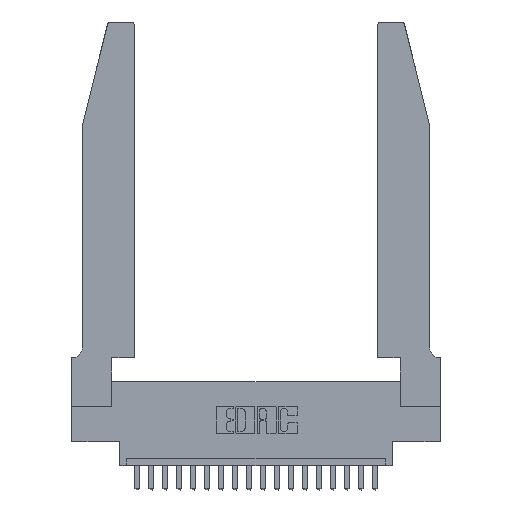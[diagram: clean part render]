
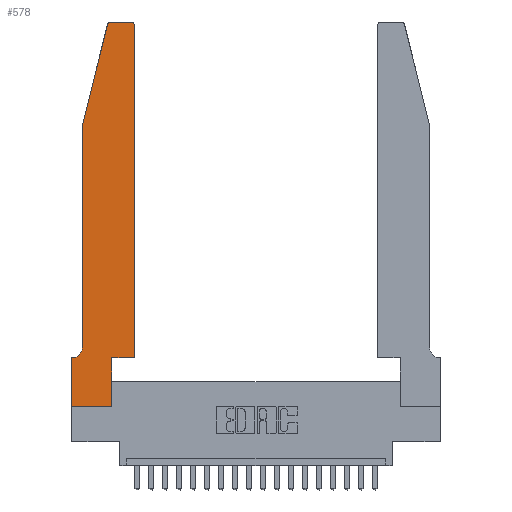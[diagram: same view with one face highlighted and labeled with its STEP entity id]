
A CAD part, top view. The second image highlights one B-rep face of the part: STEP entity #578.
In plain terms, the highlighted planar face has unit normal (0, 0, 1).
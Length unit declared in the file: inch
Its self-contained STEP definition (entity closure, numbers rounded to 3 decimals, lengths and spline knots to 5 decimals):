
#219 = CARTESIAN_POINT ( 'NONE',  ( 0.25487, 2.72718, 0.37 ) ) ;
#357 = LINE ( 'NONE', #1117, #12515 ) ;
#433 = AXIS2_PLACEMENT_3D ( 'NONE', #7943, #5994, #16182 ) ;
#545 = ORIENTED_EDGE ( 'NONE', *, *, #14522, .T. ) ;
#578 = ADVANCED_FACE ( 'NONE', ( #14978 ), #3425, .T. ) ;
#1117 = CARTESIAN_POINT ( 'NONE',  ( 0., 0., 0.37 ) ) ;
#1259 = DIRECTION ( 'NONE',  ( 1., 0., 0. ) ) ;
#1441 = LINE ( 'NONE', #11707, #9361 ) ;
#1527 = EDGE_CURVE ( 'NONE', #6507, #6493, #13141, .T. ) ;
#1722 = CARTESIAN_POINT ( 'NONE',  ( 0., 0.35, 0.37 ) ) ;
#2062 = EDGE_CURVE ( 'NONE', #17712, #14820, #6023, .T. ) ;
#2154 = ORIENTED_EDGE ( 'NONE', *, *, #14371, .T. ) ;
#2862 = CARTESIAN_POINT ( 'NONE',  ( 0.0755, 2., 0.37 ) ) ;
#3166 = VERTEX_POINT ( 'NONE', #11669 ) ;
#3185 = LINE ( 'NONE', #8729, #4270 ) ;
#3213 = CARTESIAN_POINT ( 'NONE',  ( 0.0055, 0.35, 0.37 ) ) ;
#3301 = VECTOR ( 'NONE', #17270, 39.37008 ) ;
#3425 = PLANE ( 'NONE',  #14117 ) ;
#3438 = CARTESIAN_POINT ( 'NONE',  ( 0.284, 2.75, 0.37 ) ) ;
#4258 = CARTESIAN_POINT ( 'NONE',  ( 0.2865, 0.35, 0.37 ) ) ;
#4270 = VECTOR ( 'NONE', #5372, 39.37008 ) ;
#4345 = CIRCLE ( 'NONE', #5664, 0.03 ) ;
#4473 = EDGE_CURVE ( 'NONE', #18736, #21547, #16143, .T. ) ;
#4990 = AXIS2_PLACEMENT_3D ( 'NONE', #19107, #9025, #14193 ) ;
#5372 = DIRECTION ( 'NONE',  ( -1., 0., 0. ) ) ;
#5415 = CIRCLE ( 'NONE', #433, 0.03 ) ;
#5664 = AXIS2_PLACEMENT_3D ( 'NONE', #18435, #11896, #11679 ) ;
#5994 = DIRECTION ( 'NONE',  ( 0., 0., 1. ) ) ;
#6023 = LINE ( 'NONE', #7104, #6530 ) ;
#6199 = VECTOR ( 'NONE', #21669, 39.37008 ) ;
#6493 = VERTEX_POINT ( 'NONE', #3438 ) ;
#6507 = VERTEX_POINT ( 'NONE', #8359 ) ;
#6530 = VECTOR ( 'NONE', #8620, 39.37008 ) ;
#7104 = CARTESIAN_POINT ( 'NONE',  ( 0., 0., 0.37 ) ) ;
#7943 = CARTESIAN_POINT ( 'NONE',  ( 0.4205, 2.72, 0.37 ) ) ;
#8066 = ORIENTED_EDGE ( 'NONE', *, *, #1527, .T. ) ;
#8359 = CARTESIAN_POINT ( 'NONE',  ( 0.4205, 2.75, 0.37 ) ) ;
#8620 = DIRECTION ( 'NONE',  ( 0., -1., 0. ) ) ;
#8729 = CARTESIAN_POINT ( 'NONE',  ( 0.0755, 0.35, 0.37 ) ) ;
#8849 = CARTESIAN_POINT ( 'NONE',  ( 0.4505, 2.72, 0.37 ) ) ;
#9025 = DIRECTION ( 'NONE',  ( 0., 0., -1. ) ) ;
#9279 = CARTESIAN_POINT ( 'NONE',  ( 0., 0.35, 0.37 ) ) ;
#9361 = VECTOR ( 'NONE', #16921, 39.37008 ) ;
#9556 = EDGE_CURVE ( 'NONE', #14820, #3166, #357, .T. ) ;
#9739 = CARTESIAN_POINT ( 'NONE',  ( 0.0755, 0.42, 0.37 ) ) ;
#10490 = EDGE_CURVE ( 'NONE', #3166, #19087, #17980, .T. ) ;
#10884 = ORIENTED_EDGE ( 'NONE', *, *, #9556, .T. ) ;
#11134 = EDGE_CURVE ( 'NONE', #16157, #17712, #3185, .T. ) ;
#11175 = ORIENTED_EDGE ( 'NONE', *, *, #10490, .T. ) ;
#11428 = VECTOR ( 'NONE', #13667, 39.37008 ) ;
#11669 = CARTESIAN_POINT ( 'NONE',  ( 0.2865, 0., 0.37 ) ) ;
#11679 = DIRECTION ( 'NONE',  ( 1., 0., 0. ) ) ;
#11707 = CARTESIAN_POINT ( 'NONE',  ( 0.0755, 2., 0.37 ) ) ;
#11896 = DIRECTION ( 'NONE',  ( 0., 0., 1. ) ) ;
#12056 = DIRECTION ( 'NONE',  ( 0., 0., 1. ) ) ;
#12515 = VECTOR ( 'NONE', #1259, 39.37008 ) ;
#13123 = VERTEX_POINT ( 'NONE', #15431 ) ;
#13141 = LINE ( 'NONE', #16839, #21507 ) ;
#13469 = EDGE_CURVE ( 'NONE', #19087, #13123, #17293, .T. ) ;
#13587 = ORIENTED_EDGE ( 'NONE', *, *, #17698, .T. ) ;
#13600 = DIRECTION ( 'NONE',  ( 0., 1., 0. ) ) ;
#13601 = DIRECTION ( 'NONE',  ( -1., 0., 0. ) ) ;
#13629 = ORIENTED_EDGE ( 'NONE', *, *, #4473, .T. ) ;
#13667 = DIRECTION ( 'NONE',  ( 0., -1., 0. ) ) ;
#14117 = AXIS2_PLACEMENT_3D ( 'NONE', #1722, #12056, #15258 ) ;
#14163 = VERTEX_POINT ( 'NONE', #8849 ) ;
#14193 = DIRECTION ( 'NONE',  ( -1., 0., 0. ) ) ;
#14236 = CARTESIAN_POINT ( 'NONE',  ( 0.0755, 2., 0.37 ) ) ;
#14371 = EDGE_CURVE ( 'NONE', #21218, #18736, #1441, .T. ) ;
#14459 = CARTESIAN_POINT ( 'NONE',  ( 0.4505, 0.35, 0.37 ) ) ;
#14522 = EDGE_CURVE ( 'NONE', #13123, #14163, #17528, .T. ) ;
#14567 = VECTOR ( 'NONE', #13600, 39.37008 ) ;
#14820 = VERTEX_POINT ( 'NONE', #15528 ) ;
#14978 = FACE_OUTER_BOUND ( 'NONE', #19914, .T. ) ;
#15122 = EDGE_CURVE ( 'NONE', #6493, #21218, #4345, .T. ) ;
#15250 = ORIENTED_EDGE ( 'NONE', *, *, #11134, .T. ) ;
#15258 = DIRECTION ( 'NONE',  ( 1., 0., 0. ) ) ;
#15431 = CARTESIAN_POINT ( 'NONE',  ( 0.4505, 0.35, 0.37 ) ) ;
#15507 = CARTESIAN_POINT ( 'NONE',  ( 0.2865, 0.35, 0.37 ) ) ;
#15528 = CARTESIAN_POINT ( 'NONE',  ( 0., 0., 0.37 ) ) ;
#15912 = ORIENTED_EDGE ( 'NONE', *, *, #13469, .T. ) ;
#16143 = LINE ( 'NONE', #14236, #11428 ) ;
#16157 = VERTEX_POINT ( 'NONE', #3213 ) ;
#16182 = DIRECTION ( 'NONE',  ( 1., 0., 0. ) ) ;
#16618 = ORIENTED_EDGE ( 'NONE', *, *, #2062, .T. ) ;
#16839 = CARTESIAN_POINT ( 'NONE',  ( 0.2605, 2.75, 0.37 ) ) ;
#16921 = DIRECTION ( 'NONE',  ( -0.239, -0.971, 0. ) ) ;
#17270 = DIRECTION ( 'NONE',  ( 1., 0., 0. ) ) ;
#17293 = LINE ( 'NONE', #14459, #3301 ) ;
#17528 = LINE ( 'NONE', #21525, #6199 ) ;
#17633 = ORIENTED_EDGE ( 'NONE', *, *, #20854, .T. ) ;
#17698 = EDGE_CURVE ( 'NONE', #14163, #6507, #5415, .T. ) ;
#17712 = VERTEX_POINT ( 'NONE', #9279 ) ;
#17980 = LINE ( 'NONE', #15507, #14567 ) ;
#18435 = CARTESIAN_POINT ( 'NONE',  ( 0.284, 2.72, 0.37 ) ) ;
#18736 = VERTEX_POINT ( 'NONE', #2862 ) ;
#19087 = VERTEX_POINT ( 'NONE', #4258 ) ;
#19107 = CARTESIAN_POINT ( 'NONE',  ( 0.0055, 0.42, 0.37 ) ) ;
#19500 = CIRCLE ( 'NONE', #4990, 0.07 ) ;
#19914 = EDGE_LOOP ( 'NONE', ( #8066, #20028, #2154, #13629, #17633, #15250, #16618, #10884, #11175, #15912, #545, #13587 ) ) ;
#20028 = ORIENTED_EDGE ( 'NONE', *, *, #15122, .T. ) ;
#20854 = EDGE_CURVE ( 'NONE', #21547, #16157, #19500, .T. ) ;
#21218 = VERTEX_POINT ( 'NONE', #219 ) ;
#21507 = VECTOR ( 'NONE', #13601, 39.37008 ) ;
#21525 = CARTESIAN_POINT ( 'NONE',  ( 0.4505, 0.35, 0.37 ) ) ;
#21547 = VERTEX_POINT ( 'NONE', #9739 ) ;
#21669 = DIRECTION ( 'NONE',  ( 0., 1., 0. ) ) ;
